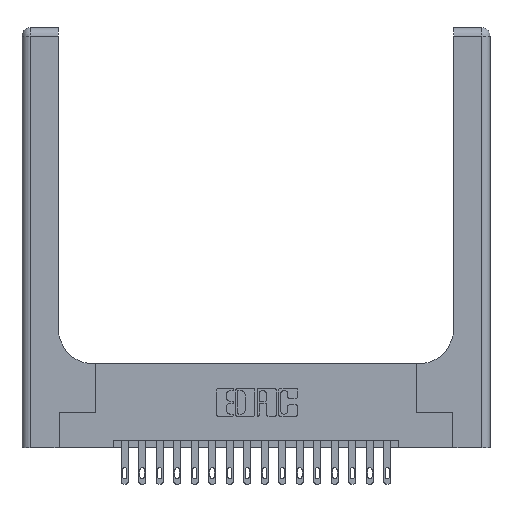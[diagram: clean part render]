
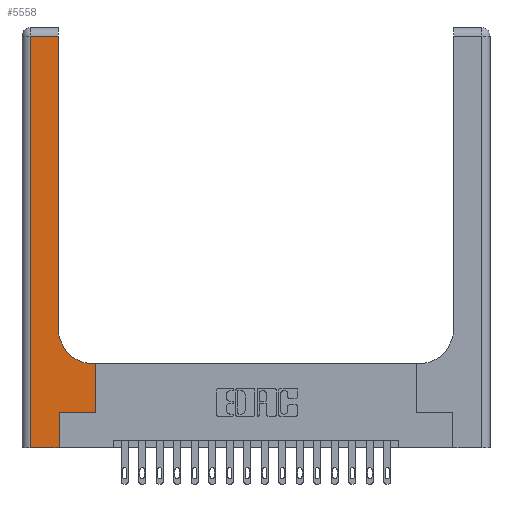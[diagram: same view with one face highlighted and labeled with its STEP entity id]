
A CAD part, top view. The second image highlights one B-rep face of the part: STEP entity #5558.
In plain terms, the highlighted planar face has unit normal (0, 0, 1).
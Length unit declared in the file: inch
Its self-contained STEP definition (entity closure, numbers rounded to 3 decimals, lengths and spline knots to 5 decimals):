
#49 = CARTESIAN_POINT ( 'NONE',  ( 0., 0., 0.37 ) ) ;
#351 = CARTESIAN_POINT ( 'NONE',  ( 0.528, 0.25, 0.37 ) ) ;
#396 = DIRECTION ( 'NONE',  ( 0., -1., 0. ) ) ;
#579 = CARTESIAN_POINT ( 'NONE',  ( 0.06, 3., 0.37 ) ) ;
#793 = DIRECTION ( 'NONE',  ( 0., 0., -1. ) ) ;
#801 = VECTOR ( 'NONE', #3780, 39.37008 ) ;
#825 = LINE ( 'NONE', #3880, #801 ) ;
#1048 = ORIENTED_EDGE ( 'NONE', *, *, #2465, .T. ) ;
#1309 = ORIENTED_EDGE ( 'NONE', *, *, #3325, .T. ) ;
#1974 = ORIENTED_EDGE ( 'NONE', *, *, #5504, .T. ) ;
#2101 = CARTESIAN_POINT ( 'NONE',  ( 0.265, 0.25, 0.37 ) ) ;
#2361 = ORIENTED_EDGE ( 'NONE', *, *, #7888, .T. ) ;
#2465 = EDGE_CURVE ( 'NONE', #4332, #11430, #5975, .T. ) ;
#3113 = CARTESIAN_POINT ( 'NONE',  ( 0.528, 0.25, 0.37 ) ) ;
#3118 = DIRECTION ( 'NONE',  ( 0., 1., 0. ) ) ;
#3325 = EDGE_CURVE ( 'NONE', #11205, #4332, #8098, .T. ) ;
#3510 = VECTOR ( 'NONE', #396, 39.37008 ) ;
#3526 = EDGE_CURVE ( 'NONE', #13568, #16518, #13133, .T. ) ;
#3548 = EDGE_CURVE ( 'NONE', #16518, #12936, #16537, .T. ) ;
#3780 = DIRECTION ( 'NONE',  ( 1., 0., 0. ) ) ;
#3859 = VERTEX_POINT ( 'NONE', #4080 ) ;
#3880 = CARTESIAN_POINT ( 'NONE',  ( 0.265, 0.25, 0.37 ) ) ;
#3921 = VECTOR ( 'NONE', #3118, 39.37008 ) ;
#4080 = CARTESIAN_POINT ( 'NONE',  ( 0.26, 2.94, 0.37 ) ) ;
#4128 = AXIS2_PLACEMENT_3D ( 'NONE', #17288, #793, #11578 ) ;
#4332 = VERTEX_POINT ( 'NONE', #12767 ) ;
#4394 = DIRECTION ( 'NONE',  ( -1., 0., 0. ) ) ;
#5240 = CARTESIAN_POINT ( 'NONE',  ( 0.51, 0.6, 0.37 ) ) ;
#5412 = VECTOR ( 'NONE', #17921, 39.37008 ) ;
#5504 = EDGE_CURVE ( 'NONE', #11430, #15012, #7571, .T. ) ;
#5558 = ADVANCED_FACE ( 'NONE', ( #16007 ), #17400, .F. ) ;
#5586 = VERTEX_POINT ( 'NONE', #14628 ) ;
#5975 = LINE ( 'NONE', #49, #12957 ) ;
#6072 = DIRECTION ( 'NONE',  ( 1., 0., 0. ) ) ;
#6631 = ORIENTED_EDGE ( 'NONE', *, *, #15561, .T. ) ;
#6932 = CARTESIAN_POINT ( 'NONE',  ( 0., 3., 0.37 ) ) ;
#6983 = LINE ( 'NONE', #10267, #12162 ) ;
#7336 = ORIENTED_EDGE ( 'NONE', *, *, #3526, .T. ) ;
#7469 = CARTESIAN_POINT ( 'NONE',  ( 0.26, 0.6, 0.37 ) ) ;
#7571 = LINE ( 'NONE', #18506, #8265 ) ;
#7888 = EDGE_CURVE ( 'NONE', #3859, #11205, #6983, .T. ) ;
#7937 = ORIENTED_EDGE ( 'NONE', *, *, #12394, .T. ) ;
#8098 = LINE ( 'NONE', #579, #3510 ) ;
#8265 = VECTOR ( 'NONE', #13597, 39.37008 ) ;
#8481 = ORIENTED_EDGE ( 'NONE', *, *, #18772, .T. ) ;
#8723 = DIRECTION ( 'NONE',  ( 0., 0., -1. ) ) ;
#9630 = CARTESIAN_POINT ( 'NONE',  ( 0.06, 2.94, 0.37 ) ) ;
#10156 = CIRCLE ( 'NONE', #4128, 0.25 ) ;
#10267 = CARTESIAN_POINT ( 'NONE',  ( 0., 2.94, 0.37 ) ) ;
#10550 = LINE ( 'NONE', #17845, #3921 ) ;
#10679 = CARTESIAN_POINT ( 'NONE',  ( 0.265, 0., 0.37 ) ) ;
#11205 = VERTEX_POINT ( 'NONE', #9630 ) ;
#11388 = DIRECTION ( 'NONE',  ( -1., 0., 0. ) ) ;
#11430 = VERTEX_POINT ( 'NONE', #10679 ) ;
#11578 = DIRECTION ( 'NONE',  ( 1., 0., 0. ) ) ;
#11745 = VECTOR ( 'NONE', #4394, 39.37008 ) ;
#12162 = VECTOR ( 'NONE', #13015, 39.37008 ) ;
#12394 = EDGE_CURVE ( 'NONE', #15012, #13568, #825, .T. ) ;
#12767 = CARTESIAN_POINT ( 'NONE',  ( 0.06, 0., 0.37 ) ) ;
#12936 = VERTEX_POINT ( 'NONE', #5240 ) ;
#12957 = VECTOR ( 'NONE', #6072, 39.37008 ) ;
#13015 = DIRECTION ( 'NONE',  ( -1., 0., 0. ) ) ;
#13133 = LINE ( 'NONE', #3113, #5412 ) ;
#13568 = VERTEX_POINT ( 'NONE', #351 ) ;
#13597 = DIRECTION ( 'NONE',  ( 0., 1., 0. ) ) ;
#13644 = EDGE_LOOP ( 'NONE', ( #8481, #2361, #1309, #1048, #1974, #7937, #7336, #14554, #6631 ) ) ;
#14554 = ORIENTED_EDGE ( 'NONE', *, *, #3548, .T. ) ;
#14628 = CARTESIAN_POINT ( 'NONE',  ( 0.26, 0.85, 0.37 ) ) ;
#15012 = VERTEX_POINT ( 'NONE', #2101 ) ;
#15561 = EDGE_CURVE ( 'NONE', #12936, #5586, #10156, .T. ) ;
#16007 = FACE_OUTER_BOUND ( 'NONE', #13644, .T. ) ;
#16518 = VERTEX_POINT ( 'NONE', #17893 ) ;
#16537 = LINE ( 'NONE', #7469, #11745 ) ;
#17288 = CARTESIAN_POINT ( 'NONE',  ( 0.51, 0.85, 0.37 ) ) ;
#17400 = PLANE ( 'NONE',  #19294 ) ;
#17845 = CARTESIAN_POINT ( 'NONE',  ( 0.26, 3., 0.37 ) ) ;
#17893 = CARTESIAN_POINT ( 'NONE',  ( 0.528, 0.6, 0.37 ) ) ;
#17921 = DIRECTION ( 'NONE',  ( 0., 1., 0. ) ) ;
#18506 = CARTESIAN_POINT ( 'NONE',  ( 0.265, 0., 0.37 ) ) ;
#18772 = EDGE_CURVE ( 'NONE', #5586, #3859, #10550, .T. ) ;
#19294 = AXIS2_PLACEMENT_3D ( 'NONE', #6932, #8723, #11388 ) ;
